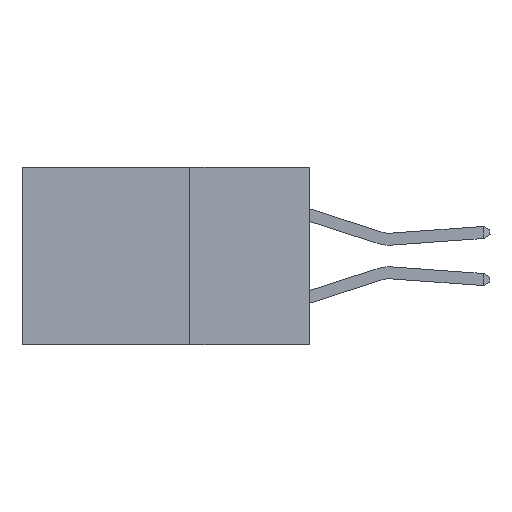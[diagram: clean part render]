
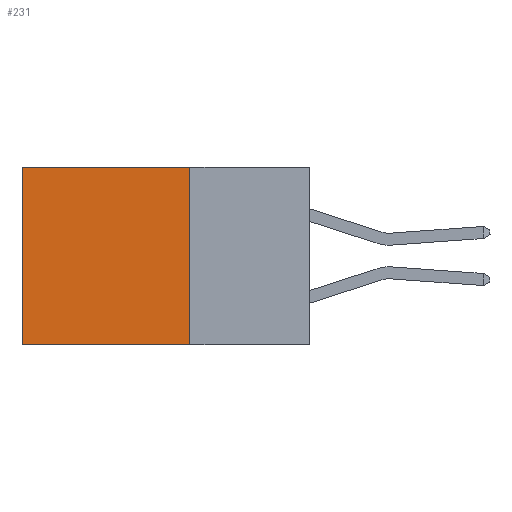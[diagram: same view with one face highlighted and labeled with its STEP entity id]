
A CAD part, left-side view. The second image highlights one B-rep face of the part: STEP entity #231.
In plain terms, the highlighted planar face has unit normal (-1, 0, 0).
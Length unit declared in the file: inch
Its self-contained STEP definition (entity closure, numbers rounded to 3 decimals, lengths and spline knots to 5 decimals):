
#188 = LINE ( 'NONE', #5234, #844 ) ;
#231 = ADVANCED_FACE ( 'NONE', ( #4788 ), #577, .F. ) ;
#530 = CARTESIAN_POINT ( 'NONE',  ( 0.2615, 0.25, 0. ) ) ;
#566 = EDGE_CURVE ( 'NONE', #10309, #6608, #9457, .T. ) ;
#577 = PLANE ( 'NONE',  #638 ) ;
#638 = AXIS2_PLACEMENT_3D ( 'NONE', #8916, #6273, #7976 ) ;
#724 = ORIENTED_EDGE ( 'NONE', *, *, #5802, .F. ) ;
#844 = VECTOR ( 'NONE', #5184, 39.37008 ) ;
#928 = DIRECTION ( 'NONE',  ( 0., 1., 0. ) ) ;
#1265 = VECTOR ( 'NONE', #2600, 39.37008 ) ;
#1357 = EDGE_CURVE ( 'NONE', #10004, #2536, #188, .T. ) ;
#1778 = CARTESIAN_POINT ( 'NONE',  ( 0.2615, 0.25, -0.37 ) ) ;
#2221 = VECTOR ( 'NONE', #4388, 39.37008 ) ;
#2327 = CARTESIAN_POINT ( 'NONE',  ( 0.2615, 0.25, -0.37 ) ) ;
#2536 = VERTEX_POINT ( 'NONE', #2327 ) ;
#2600 = DIRECTION ( 'NONE',  ( 0., 1., 0. ) ) ;
#3267 = CARTESIAN_POINT ( 'NONE',  ( 0.2615, 0.25, 0. ) ) ;
#3455 = LINE ( 'NONE', #1778, #1265 ) ;
#4288 = CARTESIAN_POINT ( 'NONE',  ( 0.2615, 0.6, -0.37 ) ) ;
#4388 = DIRECTION ( 'NONE',  ( 0., 0., -1. ) ) ;
#4788 = FACE_OUTER_BOUND ( 'NONE', #7045, .T. ) ;
#5184 = DIRECTION ( 'NONE',  ( 0., 0., -1. ) ) ;
#5234 = CARTESIAN_POINT ( 'NONE',  ( 0.2615, 0.25, -0.37 ) ) ;
#5802 = EDGE_CURVE ( 'NONE', #2536, #6608, #3455, .T. ) ;
#6273 = DIRECTION ( 'NONE',  ( 1., 0., 0. ) ) ;
#6608 = VERTEX_POINT ( 'NONE', #6696 ) ;
#6696 = CARTESIAN_POINT ( 'NONE',  ( 0.2615, 0.6, -0.37 ) ) ;
#7045 = EDGE_LOOP ( 'NONE', ( #7614, #724, #10572, #7506 ) ) ;
#7182 = VECTOR ( 'NONE', #928, 39.37008 ) ;
#7506 = ORIENTED_EDGE ( 'NONE', *, *, #9846, .T. ) ;
#7614 = ORIENTED_EDGE ( 'NONE', *, *, #566, .T. ) ;
#7976 = DIRECTION ( 'NONE',  ( 0., 0., -1. ) ) ;
#8645 = CARTESIAN_POINT ( 'NONE',  ( 0.2615, 0.6, 0. ) ) ;
#8916 = CARTESIAN_POINT ( 'NONE',  ( 0.2615, 0.25, -0.37 ) ) ;
#9457 = LINE ( 'NONE', #4288, #2221 ) ;
#9846 = EDGE_CURVE ( 'NONE', #10004, #10309, #9939, .T. ) ;
#9939 = LINE ( 'NONE', #3267, #7182 ) ;
#10004 = VERTEX_POINT ( 'NONE', #530 ) ;
#10309 = VERTEX_POINT ( 'NONE', #8645 ) ;
#10572 = ORIENTED_EDGE ( 'NONE', *, *, #1357, .F. ) ;
